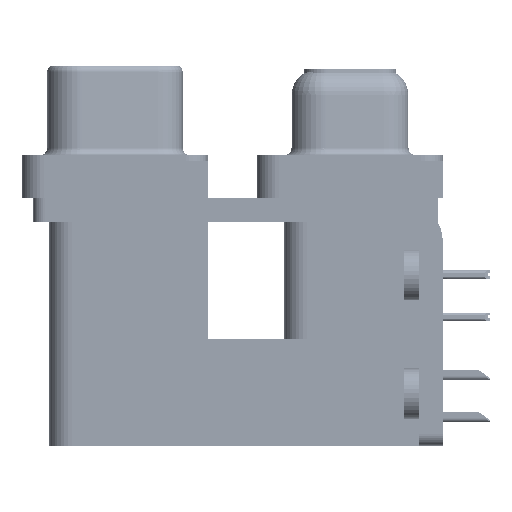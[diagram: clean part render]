
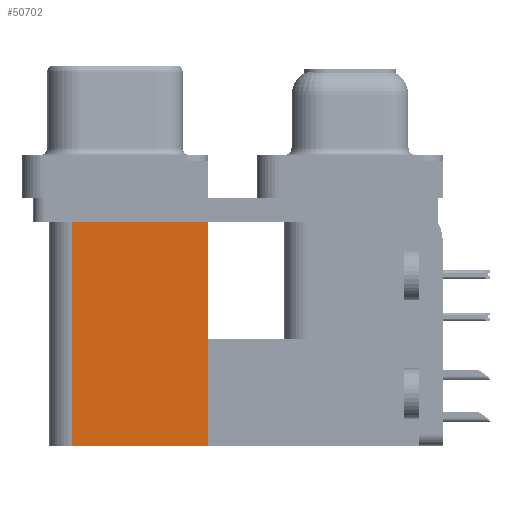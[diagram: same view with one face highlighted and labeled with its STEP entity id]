
A CAD part, left-side view. The second image highlights one B-rep face of the part: STEP entity #50702.
In plain terms, the highlighted planar face has unit normal (-1, 0, 0).
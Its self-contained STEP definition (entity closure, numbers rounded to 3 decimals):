
#115 = AXIS2_PLACEMENT_3D ( 'NONE', #27417, #16478, #1078 ) ;
#319 = CARTESIAN_POINT ( 'NONE',  ( 3.79, 9.6, -19.2 ) ) ;
#1078 = DIRECTION ( 'NONE',  ( 0., 0., -1. ) ) ;
#1900 = EDGE_LOOP ( 'NONE', ( #18031, #46228, #22417, #67264 ) ) ;
#2890 = VERTEX_POINT ( 'NONE', #21313 ) ;
#5117 = VERTEX_POINT ( 'NONE', #65296 ) ;
#5128 = DIRECTION ( 'NONE',  ( 0., 1., 0. ) ) ;
#7333 = CARTESIAN_POINT ( 'NONE',  ( 3.79, 18.8, -19.2 ) ) ;
#8667 = VERTEX_POINT ( 'NONE', #7333 ) ;
#9078 = VECTOR ( 'NONE', #52393, 1000. ) ;
#11278 = LINE ( 'NONE', #319, #50918 ) ;
#13137 = EDGE_CURVE ( 'NONE', #5117, #2890, #11278, .T. ) ;
#16478 = DIRECTION ( 'NONE',  ( 1., 0., 0. ) ) ;
#16782 = CARTESIAN_POINT ( 'NONE',  ( 3.79, 9.6, -2.5 ) ) ;
#17774 = CARTESIAN_POINT ( 'NONE',  ( 3.79, 18.8, -2.5 ) ) ;
#18031 = ORIENTED_EDGE ( 'NONE', *, *, #25705, .T. ) ;
#21313 = CARTESIAN_POINT ( 'NONE',  ( 3.79, 9.6, -2.5 ) ) ;
#22417 = ORIENTED_EDGE ( 'NONE', *, *, #23123, .F. ) ;
#23123 = EDGE_CURVE ( 'NONE', #5117, #8667, #52013, .T. ) ;
#24698 = FACE_OUTER_BOUND ( 'NONE', #1900, .T. ) ;
#25705 = EDGE_CURVE ( 'NONE', #2890, #43057, #53416, .T. ) ;
#27417 = CARTESIAN_POINT ( 'NONE',  ( 3.79, 9.6, -19.2 ) ) ;
#29609 = DIRECTION ( 'NONE',  ( 0., 0., 1. ) ) ;
#30460 = CARTESIAN_POINT ( 'NONE',  ( 3.79, 9.6, -19.2 ) ) ;
#33551 = VECTOR ( 'NONE', #29609, 1000. ) ;
#39909 = CARTESIAN_POINT ( 'NONE',  ( 3.79, 18.8, -19.2 ) ) ;
#41142 = PLANE ( 'NONE',  #115 ) ;
#43057 = VERTEX_POINT ( 'NONE', #17774 ) ;
#46228 = ORIENTED_EDGE ( 'NONE', *, *, #52726, .F. ) ;
#50170 = LINE ( 'NONE', #39909, #33551 ) ;
#50702 = ADVANCED_FACE ( 'NONE', ( #24698 ), #41142, .F. ) ;
#50918 = VECTOR ( 'NONE', #53024, 1000. ) ;
#52013 = LINE ( 'NONE', #30460, #57179 ) ;
#52393 = DIRECTION ( 'NONE',  ( 0., 1., 0. ) ) ;
#52726 = EDGE_CURVE ( 'NONE', #8667, #43057, #50170, .T. ) ;
#53024 = DIRECTION ( 'NONE',  ( 0., 0., 1. ) ) ;
#53416 = LINE ( 'NONE', #16782, #9078 ) ;
#57179 = VECTOR ( 'NONE', #5128, 1000. ) ;
#65296 = CARTESIAN_POINT ( 'NONE',  ( 3.79, 9.6, -19.2 ) ) ;
#67264 = ORIENTED_EDGE ( 'NONE', *, *, #13137, .T. ) ;
